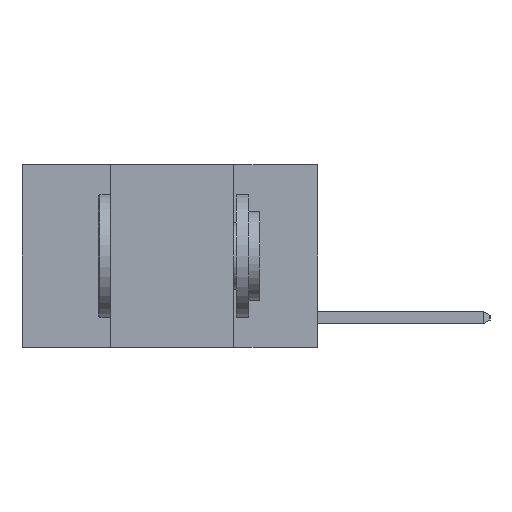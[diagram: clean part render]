
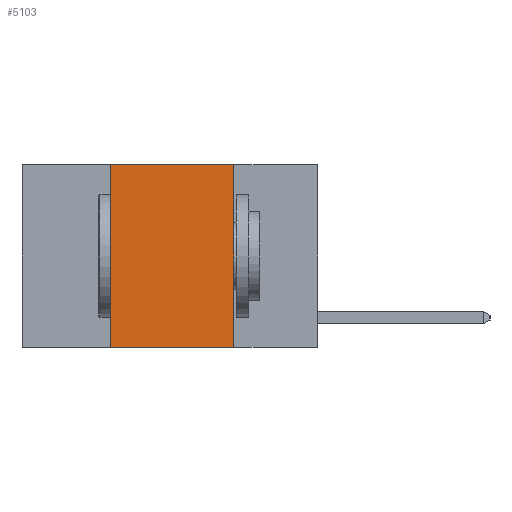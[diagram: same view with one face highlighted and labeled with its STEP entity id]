
A CAD part, left-side view. The second image highlights one B-rep face of the part: STEP entity #5103.
In plain terms, the highlighted planar face has unit normal (-1, 0, 0).
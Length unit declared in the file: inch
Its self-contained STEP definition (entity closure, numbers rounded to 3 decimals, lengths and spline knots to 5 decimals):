
#12 = ORIENTED_EDGE ( 'NONE', *, *, #3884, .F. ) ;
#797 = PLANE ( 'NONE',  #4583 ) ;
#1527 = CARTESIAN_POINT ( 'NONE',  ( 0., 0.17, 0. ) ) ;
#1595 = CARTESIAN_POINT ( 'NONE',  ( 0., 0.6, 0. ) ) ;
#1621 = LINE ( 'NONE', #1527, #9436 ) ;
#1624 = EDGE_LOOP ( 'NONE', ( #3906, #12, #2106, #4161 ) ) ;
#2106 = ORIENTED_EDGE ( 'NONE', *, *, #3380, .F. ) ;
#2130 = LINE ( 'NONE', #7195, #5998 ) ;
#2340 = DIRECTION ( 'NONE',  ( 0., 0., -1. ) ) ;
#2945 = VERTEX_POINT ( 'NONE', #4481 ) ;
#3016 = CARTESIAN_POINT ( 'NONE',  ( 0., 0.42, 0. ) ) ;
#3347 = CARTESIAN_POINT ( 'NONE',  ( 0., 0.6, -0.37 ) ) ;
#3380 = EDGE_CURVE ( 'NONE', #2945, #6720, #4694, .T. ) ;
#3884 = EDGE_CURVE ( 'NONE', #6720, #6883, #2130, .T. ) ;
#3906 = ORIENTED_EDGE ( 'NONE', *, *, #6764, .F. ) ;
#3931 = CARTESIAN_POINT ( 'NONE',  ( 0., 0.17, 0. ) ) ;
#4043 = FACE_OUTER_BOUND ( 'NONE', #1624, .T. ) ;
#4102 = VERTEX_POINT ( 'NONE', #5186 ) ;
#4161 = ORIENTED_EDGE ( 'NONE', *, *, #5820, .T. ) ;
#4481 = CARTESIAN_POINT ( 'NONE',  ( 0., 0.42, -0.37 ) ) ;
#4583 = AXIS2_PLACEMENT_3D ( 'NONE', #1595, #6936, #2340 ) ;
#4694 = LINE ( 'NONE', #8899, #8458 ) ;
#5103 = ADVANCED_FACE ( 'NONE', ( #4043 ), #797, .F. ) ;
#5164 = DIRECTION ( 'NONE',  ( 0., 0., 1. ) ) ;
#5186 = CARTESIAN_POINT ( 'NONE',  ( 0., 0.17, -0.37 ) ) ;
#5820 = EDGE_CURVE ( 'NONE', #2945, #4102, #7478, .T. ) ;
#5998 = VECTOR ( 'NONE', #7954, 39.37008 ) ;
#6720 = VERTEX_POINT ( 'NONE', #3016 ) ;
#6764 = EDGE_CURVE ( 'NONE', #6883, #4102, #1621, .T. ) ;
#6883 = VERTEX_POINT ( 'NONE', #3931 ) ;
#6936 = DIRECTION ( 'NONE',  ( 1., 0., 0. ) ) ;
#7195 = CARTESIAN_POINT ( 'NONE',  ( 0., 0.6, 0. ) ) ;
#7478 = LINE ( 'NONE', #3347, #9683 ) ;
#7621 = DIRECTION ( 'NONE',  ( 0., 0., -1. ) ) ;
#7954 = DIRECTION ( 'NONE',  ( 0., -1., 0. ) ) ;
#8458 = VECTOR ( 'NONE', #5164, 39.37008 ) ;
#8654 = DIRECTION ( 'NONE',  ( 0., -1., 0. ) ) ;
#8899 = CARTESIAN_POINT ( 'NONE',  ( 0., 0.42, 0. ) ) ;
#9436 = VECTOR ( 'NONE', #7621, 39.37008 ) ;
#9683 = VECTOR ( 'NONE', #8654, 39.37008 ) ;
